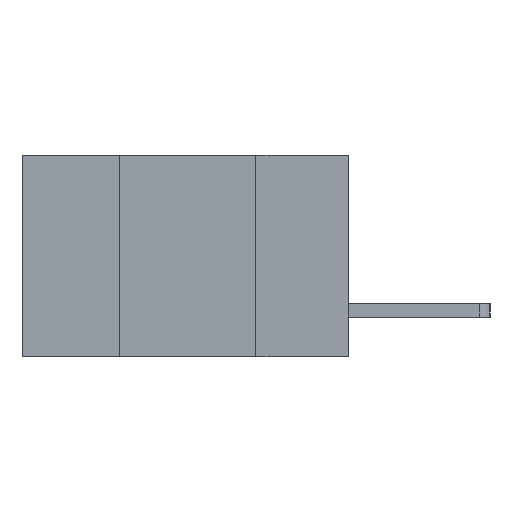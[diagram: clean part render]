
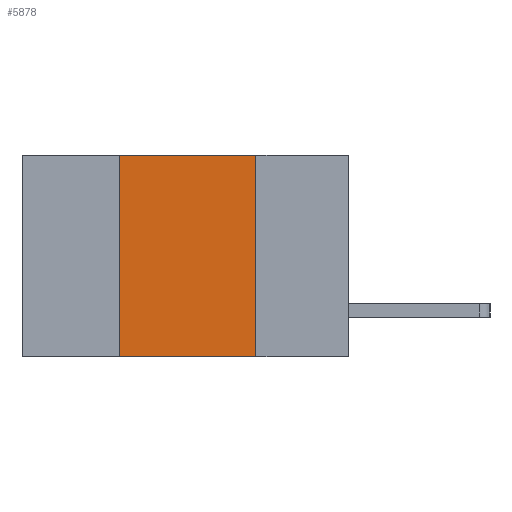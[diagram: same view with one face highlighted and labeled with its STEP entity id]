
A CAD part, left-side view. The second image highlights one B-rep face of the part: STEP entity #5878.
In plain terms, the highlighted planar face has unit normal (-1, 0, 0).
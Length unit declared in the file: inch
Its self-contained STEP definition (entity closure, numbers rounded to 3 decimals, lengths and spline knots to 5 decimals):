
#143 = CARTESIAN_POINT ( 'NONE',  ( 0., 0.17, -0.37 ) ) ;
#788 = LINE ( 'NONE', #1892, #4029 ) ;
#850 = EDGE_CURVE ( 'NONE', #5786, #8029, #2424, .T. ) ;
#1013 = ORIENTED_EDGE ( 'NONE', *, *, #7668, .T. ) ;
#1093 = CARTESIAN_POINT ( 'NONE',  ( 0., 0.42, -0.37 ) ) ;
#1300 = VECTOR ( 'NONE', #6133, 39.37008 ) ;
#1611 = CARTESIAN_POINT ( 'NONE',  ( 0., 0.6, 0. ) ) ;
#1892 = CARTESIAN_POINT ( 'NONE',  ( 0., 0.6, -0.37 ) ) ;
#2117 = VERTEX_POINT ( 'NONE', #4033 ) ;
#2424 = LINE ( 'NONE', #5073, #2616 ) ;
#2616 = VECTOR ( 'NONE', #6321, 39.37008 ) ;
#3007 = LINE ( 'NONE', #1611, #1300 ) ;
#3153 = PLANE ( 'NONE',  #5307 ) ;
#3798 = DIRECTION ( 'NONE',  ( 1., 0., 0. ) ) ;
#4029 = VECTOR ( 'NONE', #4482, 39.37008 ) ;
#4033 = CARTESIAN_POINT ( 'NONE',  ( 0., 0.17, 0. ) ) ;
#4189 = EDGE_LOOP ( 'NONE', ( #4552, #4643, #4379, #1013 ) ) ;
#4275 = EDGE_CURVE ( 'NONE', #8029, #2117, #3007, .T. ) ;
#4379 = ORIENTED_EDGE ( 'NONE', *, *, #850, .F. ) ;
#4482 = DIRECTION ( 'NONE',  ( 0., -1., 0. ) ) ;
#4552 = ORIENTED_EDGE ( 'NONE', *, *, #5705, .F. ) ;
#4643 = ORIENTED_EDGE ( 'NONE', *, *, #4275, .F. ) ;
#4783 = VECTOR ( 'NONE', #7448, 39.37008 ) ;
#4856 = VERTEX_POINT ( 'NONE', #143 ) ;
#5073 = CARTESIAN_POINT ( 'NONE',  ( 0., 0.42, -0.37 ) ) ;
#5307 = AXIS2_PLACEMENT_3D ( 'NONE', #7662, #3798, #8348 ) ;
#5536 = CARTESIAN_POINT ( 'NONE',  ( 0., 0.17, -0.37 ) ) ;
#5613 = CARTESIAN_POINT ( 'NONE',  ( 0., 0.42, 0. ) ) ;
#5705 = EDGE_CURVE ( 'NONE', #2117, #4856, #8224, .T. ) ;
#5786 = VERTEX_POINT ( 'NONE', #1093 ) ;
#5878 = ADVANCED_FACE ( 'NONE', ( #6583 ), #3153, .F. ) ;
#6133 = DIRECTION ( 'NONE',  ( 0., -1., 0. ) ) ;
#6321 = DIRECTION ( 'NONE',  ( 0., 0., 1. ) ) ;
#6583 = FACE_OUTER_BOUND ( 'NONE', #4189, .T. ) ;
#7448 = DIRECTION ( 'NONE',  ( 0., 0., -1. ) ) ;
#7662 = CARTESIAN_POINT ( 'NONE',  ( 0., 0.6, 0. ) ) ;
#7668 = EDGE_CURVE ( 'NONE', #5786, #4856, #788, .T. ) ;
#8029 = VERTEX_POINT ( 'NONE', #5613 ) ;
#8224 = LINE ( 'NONE', #5536, #4783 ) ;
#8348 = DIRECTION ( 'NONE',  ( 0., 0., -1. ) ) ;
